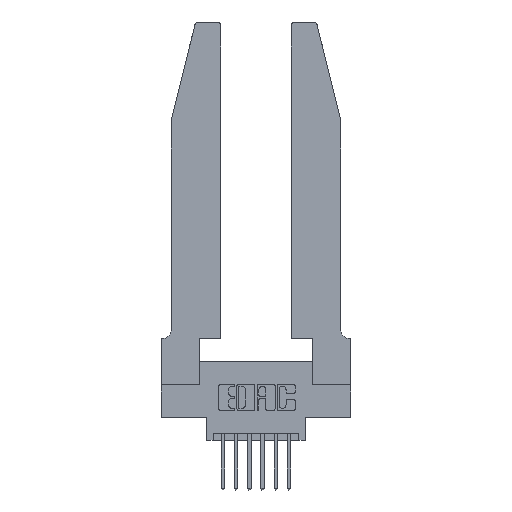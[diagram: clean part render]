
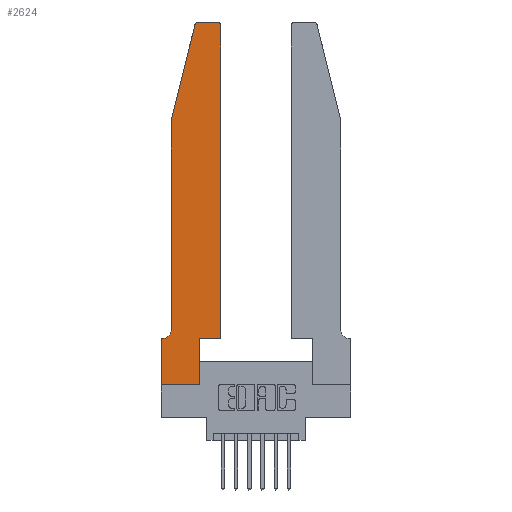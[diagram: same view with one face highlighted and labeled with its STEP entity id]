
A CAD part, top view. The second image highlights one B-rep face of the part: STEP entity #2624.
In plain terms, the highlighted planar face has unit normal (0, 0, 1).
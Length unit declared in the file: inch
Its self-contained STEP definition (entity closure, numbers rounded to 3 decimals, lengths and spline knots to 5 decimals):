
#23 = EDGE_CURVE ( 'NONE', #6572, #1337, #11063, .T. ) ;
#51 = EDGE_CURVE ( 'NONE', #1337, #10411, #4187, .T. ) ;
#276 = VERTEX_POINT ( 'NONE', #8590 ) ;
#284 = CARTESIAN_POINT ( 'NONE',  ( 0.284, 2.75, 0.37 ) ) ;
#456 = ORIENTED_EDGE ( 'NONE', *, *, #509, .T. ) ;
#509 = EDGE_CURVE ( 'NONE', #2015, #2335, #9120, .T. ) ;
#512 = DIRECTION ( 'NONE',  ( 0., -1., 0. ) ) ;
#746 = DIRECTION ( 'NONE',  ( 0., 0., 1. ) ) ;
#854 = LINE ( 'NONE', #1261, #5560 ) ;
#909 = EDGE_CURVE ( 'NONE', #5044, #13534, #2425, .T. ) ;
#920 = AXIS2_PLACEMENT_3D ( 'NONE', #930, #746, #8774 ) ;
#930 = CARTESIAN_POINT ( 'NONE',  ( 0., 0.35, 0.37 ) ) ;
#988 = FACE_OUTER_BOUND ( 'NONE', #8267, .T. ) ;
#1087 = DIRECTION ( 'NONE',  ( 1., 0., 0. ) ) ;
#1140 = CARTESIAN_POINT ( 'NONE',  ( 0.2865, 0.35, 0.37 ) ) ;
#1224 = VECTOR ( 'NONE', #4873, 39.37008 ) ;
#1261 = CARTESIAN_POINT ( 'NONE',  ( 0.2605, 2.75, 0.37 ) ) ;
#1272 = EDGE_CURVE ( 'NONE', #2335, #6229, #854, .T. ) ;
#1337 = VERTEX_POINT ( 'NONE', #3601 ) ;
#1362 = CARTESIAN_POINT ( 'NONE',  ( 0.4205, 2.72, 0.37 ) ) ;
#1661 = CARTESIAN_POINT ( 'NONE',  ( 0.4505, 0.35, 0.37 ) ) ;
#1946 = CARTESIAN_POINT ( 'NONE',  ( 0.0055, 0.35, 0.37 ) ) ;
#2015 = VERTEX_POINT ( 'NONE', #11762 ) ;
#2016 = DIRECTION ( 'NONE',  ( 0., -1., 0. ) ) ;
#2178 = ORIENTED_EDGE ( 'NONE', *, *, #12169, .T. ) ;
#2335 = VERTEX_POINT ( 'NONE', #11054 ) ;
#2350 = AXIS2_PLACEMENT_3D ( 'NONE', #8150, #2550, #11596 ) ;
#2373 = EDGE_CURVE ( 'NONE', #13534, #6572, #13252, .T. ) ;
#2425 = LINE ( 'NONE', #6390, #5043 ) ;
#2550 = DIRECTION ( 'NONE',  ( 0., 0., -1. ) ) ;
#2624 = ADVANCED_FACE ( 'NONE', ( #988 ), #14229, .T. ) ;
#3187 = ORIENTED_EDGE ( 'NONE', *, *, #7781, .T. ) ;
#3328 = ORIENTED_EDGE ( 'NONE', *, *, #2373, .T. ) ;
#3601 = CARTESIAN_POINT ( 'NONE',  ( 0.2865, 0., 0.37 ) ) ;
#3798 = CIRCLE ( 'NONE', #2350, 0.07 ) ;
#3908 = VECTOR ( 'NONE', #11796, 39.37008 ) ;
#4187 = LINE ( 'NONE', #1140, #5588 ) ;
#4210 = EDGE_CURVE ( 'NONE', #10411, #276, #11046, .T. ) ;
#4298 = VECTOR ( 'NONE', #512, 39.37008 ) ;
#4873 = DIRECTION ( 'NONE',  ( 1., 0., 0. ) ) ;
#4892 = VERTEX_POINT ( 'NONE', #8425 ) ;
#4983 = CARTESIAN_POINT ( 'NONE',  ( 0.4505, 0.35, 0.37 ) ) ;
#5043 = VECTOR ( 'NONE', #8841, 39.37008 ) ;
#5044 = VERTEX_POINT ( 'NONE', #1946 ) ;
#5305 = DIRECTION ( 'NONE',  ( -0.239, -0.971, 0. ) ) ;
#5560 = VECTOR ( 'NONE', #6788, 39.37008 ) ;
#5588 = VECTOR ( 'NONE', #14441, 39.37008 ) ;
#5663 = ORIENTED_EDGE ( 'NONE', *, *, #909, .T. ) ;
#6229 = VERTEX_POINT ( 'NONE', #284 ) ;
#6390 = CARTESIAN_POINT ( 'NONE',  ( 0.0755, 0.35, 0.37 ) ) ;
#6435 = CARTESIAN_POINT ( 'NONE',  ( 0., 0.35, 0.37 ) ) ;
#6528 = DIRECTION ( 'NONE',  ( 0., 0., 1. ) ) ;
#6572 = VERTEX_POINT ( 'NONE', #8506 ) ;
#6774 = EDGE_CURVE ( 'NONE', #4892, #5044, #3798, .T. ) ;
#6788 = DIRECTION ( 'NONE',  ( -1., 0., 0. ) ) ;
#6913 = VECTOR ( 'NONE', #5305, 39.37008 ) ;
#6942 = LINE ( 'NONE', #14377, #11353 ) ;
#7101 = ORIENTED_EDGE ( 'NONE', *, *, #23, .T. ) ;
#7122 = CARTESIAN_POINT ( 'NONE',  ( 0.2865, 0.35, 0.37 ) ) ;
#7165 = EDGE_CURVE ( 'NONE', #12544, #4892, #6942, .T. ) ;
#7213 = CARTESIAN_POINT ( 'NONE',  ( 0., 0., 0.37 ) ) ;
#7779 = ORIENTED_EDGE ( 'NONE', *, *, #6774, .T. ) ;
#7781 = EDGE_CURVE ( 'NONE', #13200, #12544, #10078, .T. ) ;
#7931 = DIRECTION ( 'NONE',  ( 0., 0., 1. ) ) ;
#8079 = VECTOR ( 'NONE', #1087, 39.37008 ) ;
#8150 = CARTESIAN_POINT ( 'NONE',  ( 0.0055, 0.42, 0.37 ) ) ;
#8267 = EDGE_LOOP ( 'NONE', ( #9138, #2178, #3187, #10711, #7779, #5663, #3328, #7101, #8853, #13125, #13996, #456 ) ) ;
#8425 = CARTESIAN_POINT ( 'NONE',  ( 0.0755, 0.42, 0.37 ) ) ;
#8506 = CARTESIAN_POINT ( 'NONE',  ( 0., 0., 0.37 ) ) ;
#8590 = CARTESIAN_POINT ( 'NONE',  ( 0.4505, 0.35, 0.37 ) ) ;
#8774 = DIRECTION ( 'NONE',  ( 1., 0., 0. ) ) ;
#8831 = EDGE_CURVE ( 'NONE', #276, #2015, #14063, .T. ) ;
#8841 = DIRECTION ( 'NONE',  ( -1., 0., 0. ) ) ;
#8853 = ORIENTED_EDGE ( 'NONE', *, *, #51, .T. ) ;
#9120 = CIRCLE ( 'NONE', #13108, 0.03 ) ;
#9138 = ORIENTED_EDGE ( 'NONE', *, *, #1272, .T. ) ;
#10078 = LINE ( 'NONE', #10911, #6913 ) ;
#10403 = CARTESIAN_POINT ( 'NONE',  ( 0.25487, 2.72718, 0.37 ) ) ;
#10411 = VERTEX_POINT ( 'NONE', #7122 ) ;
#10711 = ORIENTED_EDGE ( 'NONE', *, *, #7165, .T. ) ;
#10911 = CARTESIAN_POINT ( 'NONE',  ( 0.0755, 2., 0.37 ) ) ;
#11046 = LINE ( 'NONE', #1661, #1224 ) ;
#11054 = CARTESIAN_POINT ( 'NONE',  ( 0.4205, 2.75, 0.37 ) ) ;
#11063 = LINE ( 'NONE', #12248, #8079 ) ;
#11353 = VECTOR ( 'NONE', #2016, 39.37008 ) ;
#11493 = CIRCLE ( 'NONE', #12110, 0.03 ) ;
#11596 = DIRECTION ( 'NONE',  ( -1., 0., 0. ) ) ;
#11762 = CARTESIAN_POINT ( 'NONE',  ( 0.4505, 2.72, 0.37 ) ) ;
#11796 = DIRECTION ( 'NONE',  ( 0., 1., 0. ) ) ;
#12100 = CARTESIAN_POINT ( 'NONE',  ( 0.284, 2.72, 0.37 ) ) ;
#12110 = AXIS2_PLACEMENT_3D ( 'NONE', #12100, #6528, #12143 ) ;
#12143 = DIRECTION ( 'NONE',  ( 1., 0., 0. ) ) ;
#12169 = EDGE_CURVE ( 'NONE', #6229, #13200, #11493, .T. ) ;
#12248 = CARTESIAN_POINT ( 'NONE',  ( 0., 0., 0.37 ) ) ;
#12544 = VERTEX_POINT ( 'NONE', #14136 ) ;
#13108 = AXIS2_PLACEMENT_3D ( 'NONE', #1362, #7931, #13552 ) ;
#13125 = ORIENTED_EDGE ( 'NONE', *, *, #4210, .T. ) ;
#13200 = VERTEX_POINT ( 'NONE', #10403 ) ;
#13252 = LINE ( 'NONE', #7213, #4298 ) ;
#13534 = VERTEX_POINT ( 'NONE', #6435 ) ;
#13552 = DIRECTION ( 'NONE',  ( 1., 0., 0. ) ) ;
#13996 = ORIENTED_EDGE ( 'NONE', *, *, #8831, .T. ) ;
#14063 = LINE ( 'NONE', #4983, #3908 ) ;
#14136 = CARTESIAN_POINT ( 'NONE',  ( 0.0755, 2., 0.37 ) ) ;
#14229 = PLANE ( 'NONE',  #920 ) ;
#14377 = CARTESIAN_POINT ( 'NONE',  ( 0.0755, 2., 0.37 ) ) ;
#14441 = DIRECTION ( 'NONE',  ( 0., 1., 0. ) ) ;
